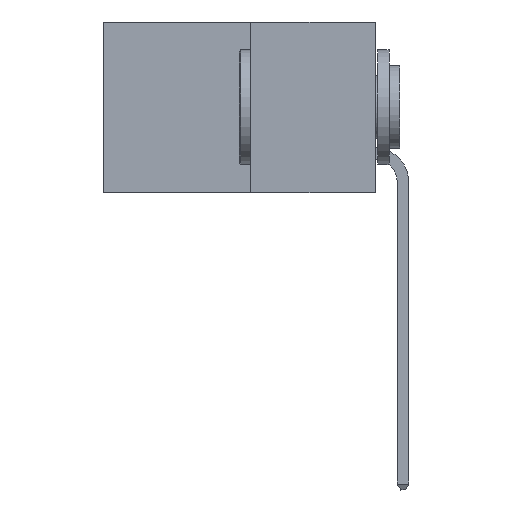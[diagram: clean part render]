
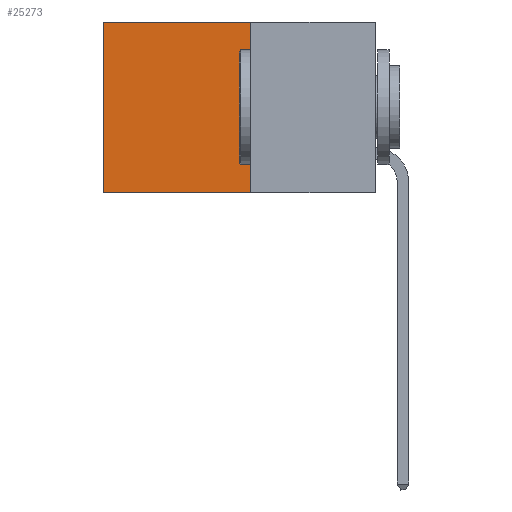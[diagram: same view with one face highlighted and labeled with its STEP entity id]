
A CAD part, left-side view. The second image highlights one B-rep face of the part: STEP entity #25273.
In plain terms, the highlighted planar face has unit normal (-1, 0, 0).
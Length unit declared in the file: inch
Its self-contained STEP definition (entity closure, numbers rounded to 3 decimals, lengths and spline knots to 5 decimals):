
#1048 = DIRECTION ( 'NONE',  ( 0., 0., -1. ) ) ;
#1555 = DIRECTION ( 'NONE',  ( 0., 0., -1. ) ) ;
#2161 = CARTESIAN_POINT ( 'NONE',  ( 0.277, 0.27, 0. ) ) ;
#3206 = LINE ( 'NONE', #16629, #26465 ) ;
#3212 = VECTOR ( 'NONE', #1048, 39.37008 ) ;
#3225 = VECTOR ( 'NONE', #3947, 39.37008 ) ;
#3707 = CARTESIAN_POINT ( 'NONE',  ( 0.277, 0.27, -0.37 ) ) ;
#3773 = FACE_OUTER_BOUND ( 'NONE', #18292, .T. ) ;
#3947 = DIRECTION ( 'NONE',  ( 0., 1., 0. ) ) ;
#5080 = CARTESIAN_POINT ( 'NONE',  ( 0.277, 0.59, -0.37 ) ) ;
#5277 = CARTESIAN_POINT ( 'NONE',  ( 0.277, 0.59, -0.37 ) ) ;
#5478 = VERTEX_POINT ( 'NONE', #5277 ) ;
#6032 = PLANE ( 'NONE',  #15729 ) ;
#6169 = CARTESIAN_POINT ( 'NONE',  ( 0.277, 0.27, -0.37 ) ) ;
#7469 = EDGE_CURVE ( 'NONE', #14114, #5478, #9291, .T. ) ;
#7751 = DIRECTION ( 'NONE',  ( 0., 0., -1. ) ) ;
#9281 = LINE ( 'NONE', #5080, #3212 ) ;
#9291 = LINE ( 'NONE', #6169, #3225 ) ;
#9688 = ORIENTED_EDGE ( 'NONE', *, *, #16262, .F. ) ;
#10564 = EDGE_CURVE ( 'NONE', #28805, #13738, #3206, .T. ) ;
#11234 = EDGE_CURVE ( 'NONE', #13738, #5478, #9281, .T. ) ;
#12111 = CARTESIAN_POINT ( 'NONE',  ( 0.277, 0.59, 0. ) ) ;
#12969 = ORIENTED_EDGE ( 'NONE', *, *, #7469, .F. ) ;
#13738 = VERTEX_POINT ( 'NONE', #12111 ) ;
#14114 = VERTEX_POINT ( 'NONE', #29171 ) ;
#14722 = ORIENTED_EDGE ( 'NONE', *, *, #11234, .T. ) ;
#15062 = LINE ( 'NONE', #27853, #24852 ) ;
#15101 = DIRECTION ( 'NONE',  ( 1., 0., 0. ) ) ;
#15729 = AXIS2_PLACEMENT_3D ( 'NONE', #3707, #15101, #1555 ) ;
#16262 = EDGE_CURVE ( 'NONE', #28805, #14114, #15062, .T. ) ;
#16629 = CARTESIAN_POINT ( 'NONE',  ( 0.277, 0.27, 0. ) ) ;
#18292 = EDGE_LOOP ( 'NONE', ( #14722, #12969, #9688, #19671 ) ) ;
#18847 = DIRECTION ( 'NONE',  ( 0., 1., 0. ) ) ;
#19671 = ORIENTED_EDGE ( 'NONE', *, *, #10564, .T. ) ;
#24852 = VECTOR ( 'NONE', #7751, 39.37008 ) ;
#25273 = ADVANCED_FACE ( 'NONE', ( #3773 ), #6032, .F. ) ;
#26465 = VECTOR ( 'NONE', #18847, 39.37008 ) ;
#27853 = CARTESIAN_POINT ( 'NONE',  ( 0.277, 0.27, -0.37 ) ) ;
#28805 = VERTEX_POINT ( 'NONE', #2161 ) ;
#29171 = CARTESIAN_POINT ( 'NONE',  ( 0.277, 0.27, -0.37 ) ) ;
